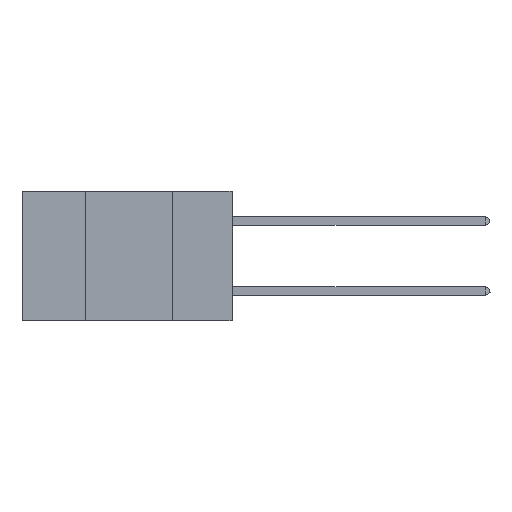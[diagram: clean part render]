
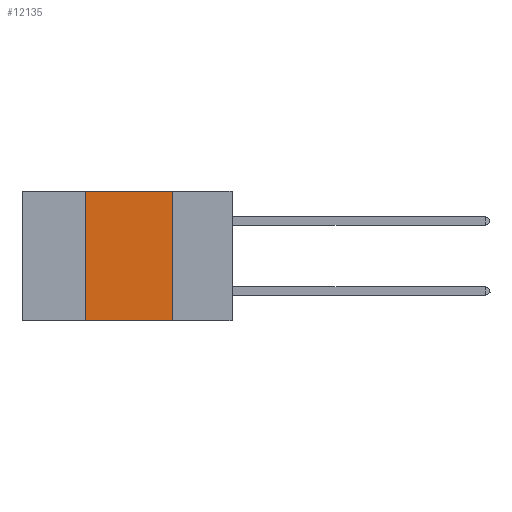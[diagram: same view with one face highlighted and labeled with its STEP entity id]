
A CAD part, left-side view. The second image highlights one B-rep face of the part: STEP entity #12135.
In plain terms, the highlighted planar face has unit normal (-1, 0, 0).
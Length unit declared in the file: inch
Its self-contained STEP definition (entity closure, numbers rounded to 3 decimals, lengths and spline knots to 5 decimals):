
#367 = ORIENTED_EDGE ( 'NONE', *, *, #4424, .F. ) ;
#401 = EDGE_CURVE ( 'NONE', #6204, #17182, #5819, .T. ) ;
#747 = VERTEX_POINT ( 'NONE', #12921 ) ;
#1869 = DIRECTION ( 'NONE',  ( 0., 0., -1. ) ) ;
#2270 = CARTESIAN_POINT ( 'NONE',  ( 0., 0.17, 0. ) ) ;
#2458 = AXIS2_PLACEMENT_3D ( 'NONE', #8327, #3721, #1869 ) ;
#2535 = CARTESIAN_POINT ( 'NONE',  ( 0., 0.42, -0.37 ) ) ;
#3721 = DIRECTION ( 'NONE',  ( 1., 0., 0. ) ) ;
#4132 = DIRECTION ( 'NONE',  ( 0., 0., -1. ) ) ;
#4424 = EDGE_CURVE ( 'NONE', #747, #17182, #17260, .T. ) ;
#4782 = CARTESIAN_POINT ( 'NONE',  ( 0., 0.42, 0. ) ) ;
#5276 = CARTESIAN_POINT ( 'NONE',  ( 0., 0.6, -0.37 ) ) ;
#5819 = LINE ( 'NONE', #5276, #7347 ) ;
#6048 = VERTEX_POINT ( 'NONE', #4782 ) ;
#6204 = VERTEX_POINT ( 'NONE', #2535 ) ;
#6853 = VECTOR ( 'NONE', #9681, 39.37008 ) ;
#7347 = VECTOR ( 'NONE', #20697, 39.37008 ) ;
#8327 = CARTESIAN_POINT ( 'NONE',  ( 0., 0.6, 0. ) ) ;
#8820 = VECTOR ( 'NONE', #4132, 39.37008 ) ;
#9681 = DIRECTION ( 'NONE',  ( 0., 0., 1. ) ) ;
#12135 = ADVANCED_FACE ( 'NONE', ( #18980 ), #19874, .F. ) ;
#12921 = CARTESIAN_POINT ( 'NONE',  ( 0., 0.17, 0. ) ) ;
#12943 = ORIENTED_EDGE ( 'NONE', *, *, #16423, .F. ) ;
#12992 = EDGE_CURVE ( 'NONE', #6048, #747, #14381, .T. ) ;
#13858 = VECTOR ( 'NONE', #19389, 39.37008 ) ;
#14381 = LINE ( 'NONE', #19524, #13858 ) ;
#15391 = EDGE_LOOP ( 'NONE', ( #367, #20831, #12943, #20812 ) ) ;
#16138 = CARTESIAN_POINT ( 'NONE',  ( 0., 0.17, -0.37 ) ) ;
#16423 = EDGE_CURVE ( 'NONE', #6204, #6048, #19831, .T. ) ;
#16468 = CARTESIAN_POINT ( 'NONE',  ( 0., 0.42, 0. ) ) ;
#17182 = VERTEX_POINT ( 'NONE', #16138 ) ;
#17260 = LINE ( 'NONE', #2270, #8820 ) ;
#18980 = FACE_OUTER_BOUND ( 'NONE', #15391, .T. ) ;
#19389 = DIRECTION ( 'NONE',  ( 0., -1., 0. ) ) ;
#19524 = CARTESIAN_POINT ( 'NONE',  ( 0., 0.6, 0. ) ) ;
#19831 = LINE ( 'NONE', #16468, #6853 ) ;
#19874 = PLANE ( 'NONE',  #2458 ) ;
#20697 = DIRECTION ( 'NONE',  ( 0., -1., 0. ) ) ;
#20812 = ORIENTED_EDGE ( 'NONE', *, *, #401, .T. ) ;
#20831 = ORIENTED_EDGE ( 'NONE', *, *, #12992, .F. ) ;
